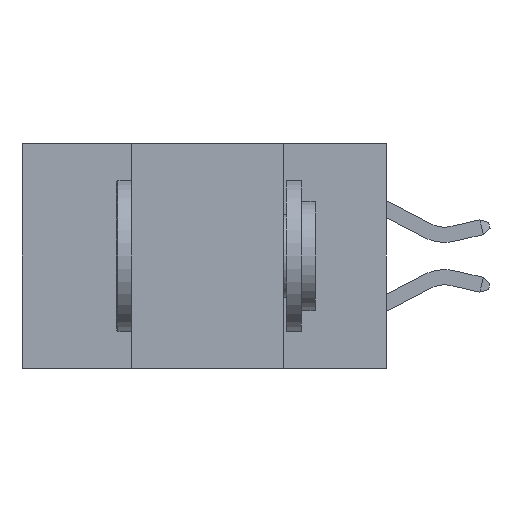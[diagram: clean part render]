
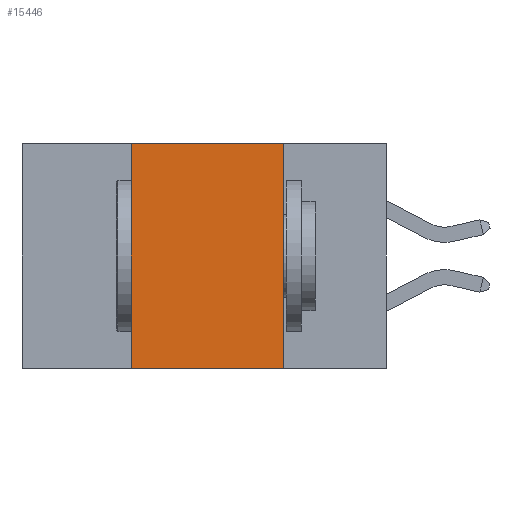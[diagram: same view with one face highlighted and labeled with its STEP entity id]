
A CAD part, left-side view. The second image highlights one B-rep face of the part: STEP entity #15446.
In plain terms, the highlighted planar face has unit normal (-1, 0, 0).
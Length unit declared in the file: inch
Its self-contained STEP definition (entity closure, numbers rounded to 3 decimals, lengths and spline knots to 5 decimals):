
#24 = LINE ( 'NONE', #25515, #5101 ) ;
#456 = VERTEX_POINT ( 'NONE', #12992 ) ;
#862 = ORIENTED_EDGE ( 'NONE', *, *, #20281, .F. ) ;
#921 = DIRECTION ( 'NONE',  ( 0., 0., -1. ) ) ;
#1030 = CARTESIAN_POINT ( 'NONE',  ( 0., 0.6, 0. ) ) ;
#1197 = CARTESIAN_POINT ( 'NONE',  ( 0., 0.17, 0. ) ) ;
#1809 = CARTESIAN_POINT ( 'NONE',  ( 0., 0.6, -0.37 ) ) ;
#1976 = AXIS2_PLACEMENT_3D ( 'NONE', #1030, #7465, #5369 ) ;
#2659 = ORIENTED_EDGE ( 'NONE', *, *, #3519, .F. ) ;
#3113 = CARTESIAN_POINT ( 'NONE',  ( 0., 0.17, -0.37 ) ) ;
#3197 = CARTESIAN_POINT ( 'NONE',  ( 0., 0.42, 0. ) ) ;
#3209 = PLANE ( 'NONE',  #1976 ) ;
#3519 = EDGE_CURVE ( 'NONE', #456, #20359, #24, .T. ) ;
#5091 = DIRECTION ( 'NONE',  ( 0., -1., 0. ) ) ;
#5101 = VECTOR ( 'NONE', #25756, 39.37008 ) ;
#5369 = DIRECTION ( 'NONE',  ( 0., 0., -1. ) ) ;
#6186 = LINE ( 'NONE', #3113, #16809 ) ;
#7266 = CARTESIAN_POINT ( 'NONE',  ( 0., 0.6, 0. ) ) ;
#7465 = DIRECTION ( 'NONE',  ( 1., 0., 0. ) ) ;
#9021 = CARTESIAN_POINT ( 'NONE',  ( 0., 0.17, -0.37 ) ) ;
#12712 = VECTOR ( 'NONE', #5091, 39.37008 ) ;
#12992 = CARTESIAN_POINT ( 'NONE',  ( 0., 0.42, -0.37 ) ) ;
#13490 = VERTEX_POINT ( 'NONE', #1197 ) ;
#15446 = ADVANCED_FACE ( 'NONE', ( #23109 ), #3209, .F. ) ;
#15819 = ORIENTED_EDGE ( 'NONE', *, *, #18326, .F. ) ;
#16727 = DIRECTION ( 'NONE',  ( 0., -1., 0. ) ) ;
#16809 = VECTOR ( 'NONE', #921, 39.37008 ) ;
#17076 = EDGE_LOOP ( 'NONE', ( #15819, #862, #2659, #20156 ) ) ;
#18326 = EDGE_CURVE ( 'NONE', #13490, #25707, #6186, .T. ) ;
#20156 = ORIENTED_EDGE ( 'NONE', *, *, #26807, .T. ) ;
#20281 = EDGE_CURVE ( 'NONE', #20359, #13490, #24605, .T. ) ;
#20359 = VERTEX_POINT ( 'NONE', #3197 ) ;
#21664 = LINE ( 'NONE', #1809, #27249 ) ;
#23109 = FACE_OUTER_BOUND ( 'NONE', #17076, .T. ) ;
#24605 = LINE ( 'NONE', #7266, #12712 ) ;
#25515 = CARTESIAN_POINT ( 'NONE',  ( 0., 0.42, -0.37 ) ) ;
#25707 = VERTEX_POINT ( 'NONE', #9021 ) ;
#25756 = DIRECTION ( 'NONE',  ( 0., 0., 1. ) ) ;
#26807 = EDGE_CURVE ( 'NONE', #456, #25707, #21664, .T. ) ;
#27249 = VECTOR ( 'NONE', #16727, 39.37008 ) ;
